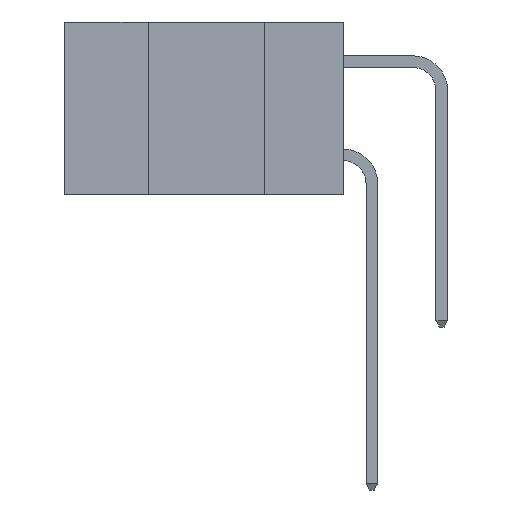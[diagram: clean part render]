
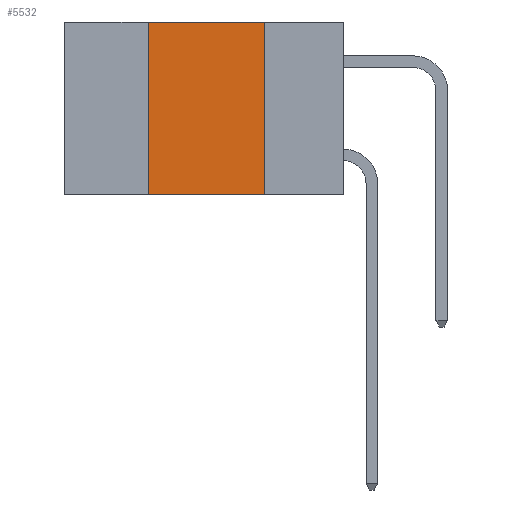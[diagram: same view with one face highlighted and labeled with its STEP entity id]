
A CAD part, left-side view. The second image highlights one B-rep face of the part: STEP entity #5532.
In plain terms, the highlighted planar face has unit normal (-1, 0, 0).
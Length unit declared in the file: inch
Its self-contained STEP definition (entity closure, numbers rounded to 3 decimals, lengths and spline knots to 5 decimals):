
#255 = VERTEX_POINT ( 'NONE', #4843 ) ;
#1551 = CARTESIAN_POINT ( 'NONE',  ( 0., 0.42, 0. ) ) ;
#2299 = ORIENTED_EDGE ( 'NONE', *, *, #2925, .F. ) ;
#2378 = CARTESIAN_POINT ( 'NONE',  ( 0., 0.42, -0.37 ) ) ;
#2902 = VERTEX_POINT ( 'NONE', #14253 ) ;
#2925 = EDGE_CURVE ( 'NONE', #2902, #14976, #13242, .T. ) ;
#3239 = VECTOR ( 'NONE', #4674, 39.37008 ) ;
#4656 = ORIENTED_EDGE ( 'NONE', *, *, #8930, .F. ) ;
#4674 = DIRECTION ( 'NONE',  ( 0., 0., 1. ) ) ;
#4843 = CARTESIAN_POINT ( 'NONE',  ( 0., 0.17, -0.37 ) ) ;
#5532 = ADVANCED_FACE ( 'NONE', ( #10517 ), #14941, .F. ) ;
#6647 = DIRECTION ( 'NONE',  ( 0., -1., 0. ) ) ;
#6694 = CARTESIAN_POINT ( 'NONE',  ( 0., 0.6, -0.37 ) ) ;
#8080 = LINE ( 'NONE', #10123, #10938 ) ;
#8299 = CARTESIAN_POINT ( 'NONE',  ( 0., 0.17, 0. ) ) ;
#8492 = VECTOR ( 'NONE', #6647, 39.37008 ) ;
#8716 = AXIS2_PLACEMENT_3D ( 'NONE', #14442, #14543, #14530 ) ;
#8930 = EDGE_CURVE ( 'NONE', #14976, #9310, #11209, .T. ) ;
#9119 = ORIENTED_EDGE ( 'NONE', *, *, #14158, .F. ) ;
#9310 = VERTEX_POINT ( 'NONE', #8299 ) ;
#9541 = EDGE_CURVE ( 'NONE', #2902, #255, #14981, .T. ) ;
#10015 = DIRECTION ( 'NONE',  ( 0., 0., -1. ) ) ;
#10123 = CARTESIAN_POINT ( 'NONE',  ( 0., 0.17, -0.37 ) ) ;
#10517 = FACE_OUTER_BOUND ( 'NONE', #14658, .T. ) ;
#10834 = VECTOR ( 'NONE', #11165, 39.37008 ) ;
#10938 = VECTOR ( 'NONE', #10015, 39.37008 ) ;
#11165 = DIRECTION ( 'NONE',  ( 0., -1., 0. ) ) ;
#11193 = CARTESIAN_POINT ( 'NONE',  ( 0., 0.6, 0. ) ) ;
#11209 = LINE ( 'NONE', #11193, #10834 ) ;
#13242 = LINE ( 'NONE', #2378, #3239 ) ;
#14158 = EDGE_CURVE ( 'NONE', #9310, #255, #8080, .T. ) ;
#14253 = CARTESIAN_POINT ( 'NONE',  ( 0., 0.42, -0.37 ) ) ;
#14442 = CARTESIAN_POINT ( 'NONE',  ( 0., 0.6, 0. ) ) ;
#14530 = DIRECTION ( 'NONE',  ( 0., 0., -1. ) ) ;
#14543 = DIRECTION ( 'NONE',  ( 1., 0., 0. ) ) ;
#14658 = EDGE_LOOP ( 'NONE', ( #9119, #4656, #2299, #14782 ) ) ;
#14782 = ORIENTED_EDGE ( 'NONE', *, *, #9541, .T. ) ;
#14941 = PLANE ( 'NONE',  #8716 ) ;
#14976 = VERTEX_POINT ( 'NONE', #1551 ) ;
#14981 = LINE ( 'NONE', #6694, #8492 ) ;
